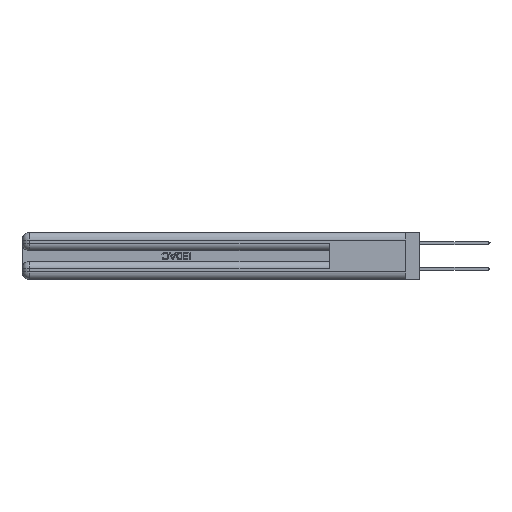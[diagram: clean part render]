
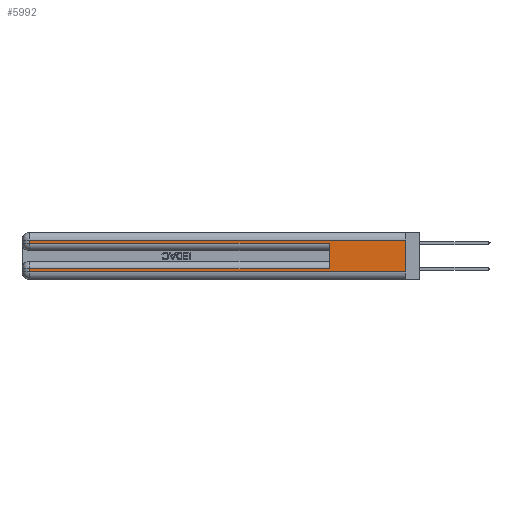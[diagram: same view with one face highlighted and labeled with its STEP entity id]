
A CAD part, left-side view. The second image highlights one B-rep face of the part: STEP entity #5992.
In plain terms, the highlighted planar face has unit normal (-1, 0, 0).
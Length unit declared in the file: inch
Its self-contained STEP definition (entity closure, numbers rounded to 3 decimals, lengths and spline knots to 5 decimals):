
#666 = EDGE_CURVE ( 'NONE', #24599, #15715, #33410, .T. ) ;
#892 = EDGE_CURVE ( 'NONE', #24599, #30314, #29444, .T. ) ;
#1923 = EDGE_CURVE ( 'NONE', #13486, #30314, #47429, .T. ) ;
#2786 = ORIENTED_EDGE ( 'NONE', *, *, #30147, .F. ) ;
#3404 = DIRECTION ( 'NONE',  ( 0., 0., -1. ) ) ;
#4135 = DIRECTION ( 'NONE',  ( 1., 0., 0. ) ) ;
#4404 = ORIENTED_EDGE ( 'NONE', *, *, #892, .F. ) ;
#5992 = ADVANCED_FACE ( 'NONE', ( #40395 ), #42380, .F. ) ;
#7474 = VECTOR ( 'NONE', #3404, 39.37008 ) ;
#8004 = CARTESIAN_POINT ( 'NONE',  ( 0., 0., 0.31 ) ) ;
#9332 = ORIENTED_EDGE ( 'NONE', *, *, #33486, .T. ) ;
#10311 = CARTESIAN_POINT ( 'NONE',  ( 0., 0.6, 0.285 ) ) ;
#12654 = CARTESIAN_POINT ( 'NONE',  ( 0., 2.94, 0.31 ) ) ;
#13136 = CARTESIAN_POINT ( 'NONE',  ( 0., 2.94, 0.37 ) ) ;
#13246 = DIRECTION ( 'NONE',  ( 0., 0., -1. ) ) ;
#13486 = VERTEX_POINT ( 'NONE', #42789 ) ;
#13495 = ORIENTED_EDGE ( 'NONE', *, *, #1923, .T. ) ;
#14060 = EDGE_LOOP ( 'NONE', ( #4404, #24431, #42103, #16149, #2786, #9332, #15448, #13495 ) ) ;
#14635 = VECTOR ( 'NONE', #24746, 39.37008 ) ;
#14691 = VECTOR ( 'NONE', #28874, 39.37008 ) ;
#15448 = ORIENTED_EDGE ( 'NONE', *, *, #25517, .T. ) ;
#15715 = VERTEX_POINT ( 'NONE', #12654 ) ;
#16149 = ORIENTED_EDGE ( 'NONE', *, *, #45858, .T. ) ;
#16213 = CARTESIAN_POINT ( 'NONE',  ( 0., 2.94, 0.085 ) ) ;
#17630 = CARTESIAN_POINT ( 'NONE',  ( 0., 0.6, 0.085 ) ) ;
#19264 = VECTOR ( 'NONE', #13246, 39.37008 ) ;
#23053 = DIRECTION ( 'NONE',  ( 0., 1., 0. ) ) ;
#23178 = VECTOR ( 'NONE', #23053, 39.37008 ) ;
#23228 = CARTESIAN_POINT ( 'NONE',  ( 0., 0., 0.37 ) ) ;
#23346 = VECTOR ( 'NONE', #46809, 39.37008 ) ;
#24431 = ORIENTED_EDGE ( 'NONE', *, *, #666, .T. ) ;
#24599 = VERTEX_POINT ( 'NONE', #36261 ) ;
#24746 = DIRECTION ( 'NONE',  ( 0., 0., -1. ) ) ;
#24757 = CARTESIAN_POINT ( 'NONE',  ( 0., 2.94, 0.285 ) ) ;
#24799 = DIRECTION ( 'NONE',  ( 0., -1., 0. ) ) ;
#24921 = LINE ( 'NONE', #25020, #14691 ) ;
#25020 = CARTESIAN_POINT ( 'NONE',  ( 0., 0.6, 0.145 ) ) ;
#25517 = EDGE_CURVE ( 'NONE', #48322, #13486, #35123, .T. ) ;
#26410 = LINE ( 'NONE', #39973, #45689 ) ;
#26556 = CARTESIAN_POINT ( 'NONE',  ( 0., 2.94, 0.37 ) ) ;
#27038 = DIRECTION ( 'NONE',  ( 0., 0., -1. ) ) ;
#28874 = DIRECTION ( 'NONE',  ( 0., 0., 1. ) ) ;
#29444 = LINE ( 'NONE', #32444, #19264 ) ;
#29700 = CARTESIAN_POINT ( 'NONE',  ( 0., 0., 0.06 ) ) ;
#30147 = EDGE_CURVE ( 'NONE', #38913, #34188, #24921, .T. ) ;
#30314 = VERTEX_POINT ( 'NONE', #29700 ) ;
#30781 = AXIS2_PLACEMENT_3D ( 'NONE', #23228, #4135, #27038 ) ;
#30790 = DIRECTION ( 'NONE',  ( 0., 1., 0. ) ) ;
#32191 = LINE ( 'NONE', #49970, #41197 ) ;
#32444 = CARTESIAN_POINT ( 'NONE',  ( 0., 0., 0.37 ) ) ;
#33410 = LINE ( 'NONE', #8004, #23178 ) ;
#33486 = EDGE_CURVE ( 'NONE', #38913, #48322, #32191, .T. ) ;
#34188 = VERTEX_POINT ( 'NONE', #10311 ) ;
#35123 = LINE ( 'NONE', #13136, #14635 ) ;
#36261 = CARTESIAN_POINT ( 'NONE',  ( 0., 0., 0.31 ) ) ;
#38221 = LINE ( 'NONE', #26556, #7474 ) ;
#38913 = VERTEX_POINT ( 'NONE', #17630 ) ;
#39086 = CARTESIAN_POINT ( 'NONE',  ( 0., 0., 0.06 ) ) ;
#39973 = CARTESIAN_POINT ( 'NONE',  ( 0., 0., 0.285 ) ) ;
#40395 = FACE_OUTER_BOUND ( 'NONE', #14060, .T. ) ;
#41197 = VECTOR ( 'NONE', #30790, 39.37008 ) ;
#42103 = ORIENTED_EDGE ( 'NONE', *, *, #48671, .T. ) ;
#42380 = PLANE ( 'NONE',  #30781 ) ;
#42789 = CARTESIAN_POINT ( 'NONE',  ( 0., 2.94, 0.06 ) ) ;
#44328 = VERTEX_POINT ( 'NONE', #24757 ) ;
#45689 = VECTOR ( 'NONE', #24799, 39.37008 ) ;
#45858 = EDGE_CURVE ( 'NONE', #44328, #34188, #26410, .T. ) ;
#46809 = DIRECTION ( 'NONE',  ( 0., -1., 0. ) ) ;
#47429 = LINE ( 'NONE', #39086, #23346 ) ;
#48322 = VERTEX_POINT ( 'NONE', #16213 ) ;
#48671 = EDGE_CURVE ( 'NONE', #15715, #44328, #38221, .T. ) ;
#49970 = CARTESIAN_POINT ( 'NONE',  ( 0., 0., 0.085 ) ) ;
